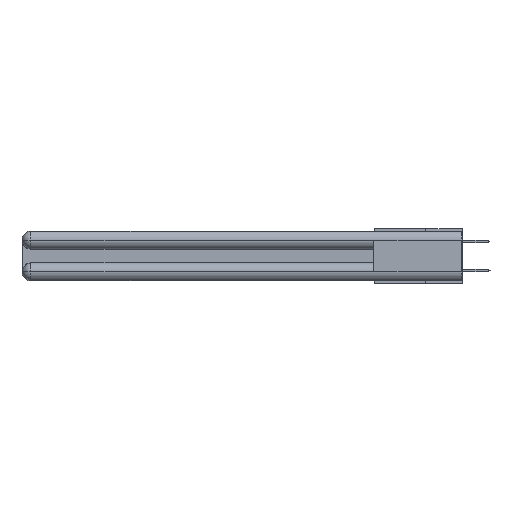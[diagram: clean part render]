
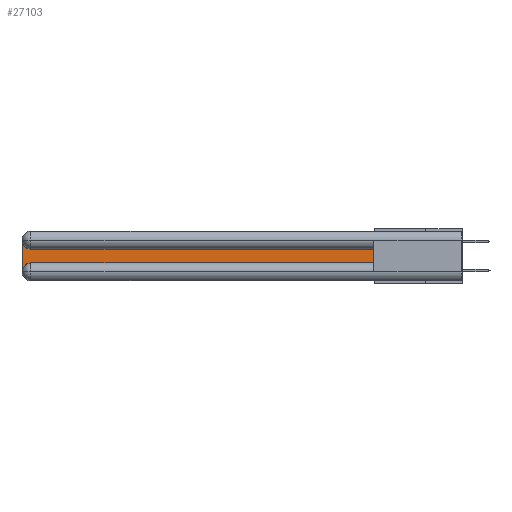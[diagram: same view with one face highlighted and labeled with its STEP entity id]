
A CAD part, left-side view. The second image highlights one B-rep face of the part: STEP entity #27103.
In plain terms, the highlighted planar face has unit normal (-1, 0, 0).
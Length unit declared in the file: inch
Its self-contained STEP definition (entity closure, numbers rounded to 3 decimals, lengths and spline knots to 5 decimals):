
#391 = DIRECTION ( 'NONE',  ( 1., 0., 0. ) ) ;
#1230 = CARTESIAN_POINT ( 'NONE',  ( 0.075, 3., -0.2175 ) ) ;
#1806 = CARTESIAN_POINT ( 'NONE',  ( 0.075, 0.6, -0.2175 ) ) ;
#2068 = AXIS2_PLACEMENT_3D ( 'NONE', #12235, #15395, #28985 ) ;
#3369 = EDGE_CURVE ( 'NONE', #16610, #11175, #3716, .T. ) ;
#3716 = LINE ( 'NONE', #31689, #18054 ) ;
#4319 = CARTESIAN_POINT ( 'NONE',  ( 0.075, 0.6, -0.1225 ) ) ;
#5341 = ORIENTED_EDGE ( 'NONE', *, *, #16605, .T. ) ;
#6447 = EDGE_CURVE ( 'NONE', #6715, #13481, #14349, .T. ) ;
#6663 = ORIENTED_EDGE ( 'NONE', *, *, #31075, .T. ) ;
#6715 = VERTEX_POINT ( 'NONE', #17461 ) ;
#6896 = CIRCLE ( 'NONE', #13186, 0.06 ) ;
#7839 = LINE ( 'NONE', #1806, #34408 ) ;
#9013 = CARTESIAN_POINT ( 'NONE',  ( 0.075, 2.94, -0.0625 ) ) ;
#10240 = DIRECTION ( 'NONE',  ( 0., 1., 0. ) ) ;
#11175 = VERTEX_POINT ( 'NONE', #4319 ) ;
#11250 = ORIENTED_EDGE ( 'NONE', *, *, #35882, .T. ) ;
#12235 = CARTESIAN_POINT ( 'NONE',  ( 0.075, 2.94, -0.2775 ) ) ;
#12538 = CARTESIAN_POINT ( 'NONE',  ( 0.075, 0.6, -0.2175 ) ) ;
#12766 = CARTESIAN_POINT ( 'NONE',  ( 0.075, 2.94, -0.1225 ) ) ;
#13186 = AXIS2_PLACEMENT_3D ( 'NONE', #9013, #391, #20054 ) ;
#13481 = VERTEX_POINT ( 'NONE', #26793 ) ;
#13766 = DIRECTION ( 'NONE',  ( 1., 0., 0. ) ) ;
#14349 = CIRCLE ( 'NONE', #2068, 0.06 ) ;
#15365 = CARTESIAN_POINT ( 'NONE',  ( 0.075, 0.6, -0.1225 ) ) ;
#15395 = DIRECTION ( 'NONE',  ( 1., 0., 0. ) ) ;
#16605 = EDGE_CURVE ( 'NONE', #13481, #16610, #7839, .T. ) ;
#16610 = VERTEX_POINT ( 'NONE', #12538 ) ;
#16675 = CARTESIAN_POINT ( 'NONE',  ( 0.075, 3., -0.0625 ) ) ;
#17461 = CARTESIAN_POINT ( 'NONE',  ( 0.075, 3., -0.2775 ) ) ;
#17890 = EDGE_CURVE ( 'NONE', #33627, #6715, #25590, .T. ) ;
#18054 = VECTOR ( 'NONE', #29250, 39.37008 ) ;
#19416 = DIRECTION ( 'NONE',  ( 0., 0., -1. ) ) ;
#20054 = DIRECTION ( 'NONE',  ( 0., 0., -1. ) ) ;
#20091 = ORIENTED_EDGE ( 'NONE', *, *, #17890, .T. ) ;
#20677 = DIRECTION ( 'NONE',  ( 0., 0., -1. ) ) ;
#20773 = AXIS2_PLACEMENT_3D ( 'NONE', #33200, #13766, #19416 ) ;
#22008 = EDGE_LOOP ( 'NONE', ( #11250, #6663, #20091, #33355, #5341, #31849 ) ) ;
#22219 = PLANE ( 'NONE',  #20773 ) ;
#25590 = LINE ( 'NONE', #1230, #28196 ) ;
#25694 = VECTOR ( 'NONE', #10240, 39.37008 ) ;
#26793 = CARTESIAN_POINT ( 'NONE',  ( 0.075, 2.94, -0.2175 ) ) ;
#27103 = ADVANCED_FACE ( 'NONE', ( #32310 ), #22219, .F. ) ;
#28196 = VECTOR ( 'NONE', #20677, 39.37008 ) ;
#28985 = DIRECTION ( 'NONE',  ( 0., 0., -1. ) ) ;
#29149 = DIRECTION ( 'NONE',  ( 0., -1., 0. ) ) ;
#29250 = DIRECTION ( 'NONE',  ( 0., 0., 1. ) ) ;
#31075 = EDGE_CURVE ( 'NONE', #34554, #33627, #6896, .T. ) ;
#31689 = CARTESIAN_POINT ( 'NONE',  ( 0.075, 0.6, -0.2175 ) ) ;
#31849 = ORIENTED_EDGE ( 'NONE', *, *, #3369, .T. ) ;
#32310 = FACE_OUTER_BOUND ( 'NONE', #22008, .T. ) ;
#33200 = CARTESIAN_POINT ( 'NONE',  ( 0.075, 3., -0.1225 ) ) ;
#33355 = ORIENTED_EDGE ( 'NONE', *, *, #6447, .T. ) ;
#33576 = LINE ( 'NONE', #15365, #25694 ) ;
#33627 = VERTEX_POINT ( 'NONE', #16675 ) ;
#34408 = VECTOR ( 'NONE', #29149, 39.37008 ) ;
#34554 = VERTEX_POINT ( 'NONE', #12766 ) ;
#35882 = EDGE_CURVE ( 'NONE', #11175, #34554, #33576, .T. ) ;
